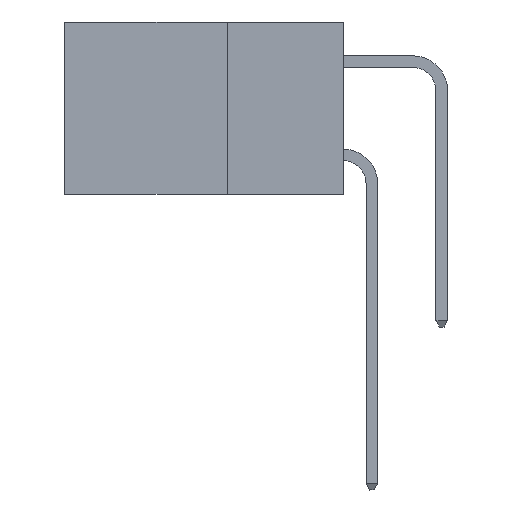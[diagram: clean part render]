
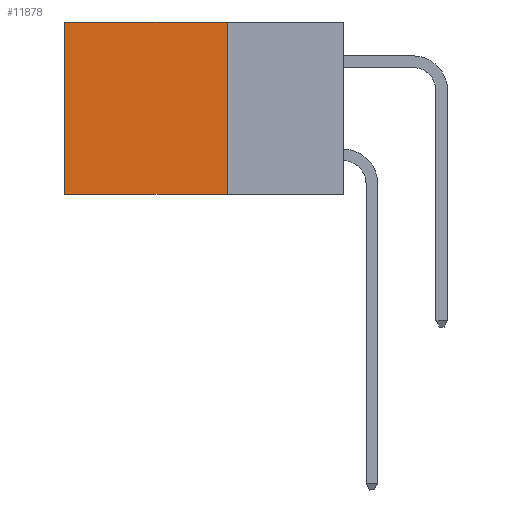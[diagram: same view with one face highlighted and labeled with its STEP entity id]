
A CAD part, left-side view. The second image highlights one B-rep face of the part: STEP entity #11878.
In plain terms, the highlighted planar face has unit normal (-1, 0, 0).
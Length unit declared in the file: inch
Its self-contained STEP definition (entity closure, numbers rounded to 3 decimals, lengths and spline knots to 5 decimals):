
#18 = LINE ( 'NONE', #16242, #24884 ) ;
#722 = ORIENTED_EDGE ( 'NONE', *, *, #7948, .F. ) ;
#1176 = EDGE_CURVE ( 'NONE', #22438, #4919, #18, .T. ) ;
#4236 = LINE ( 'NONE', #7374, #10094 ) ;
#4919 = VERTEX_POINT ( 'NONE', #7055 ) ;
#6580 = PLANE ( 'NONE',  #23420 ) ;
#6686 = CARTESIAN_POINT ( 'NONE',  ( 0.2615, 0.25, -0.37 ) ) ;
#7055 = CARTESIAN_POINT ( 'NONE',  ( 0.2615, 0.6, 0. ) ) ;
#7374 = CARTESIAN_POINT ( 'NONE',  ( 0.2615, 0.25, -0.37 ) ) ;
#7934 = VECTOR ( 'NONE', #24106, 39.37008 ) ;
#7948 = EDGE_CURVE ( 'NONE', #22438, #12869, #22964, .T. ) ;
#8072 = EDGE_CURVE ( 'NONE', #12869, #18795, #4236, .T. ) ;
#9987 = EDGE_LOOP ( 'NONE', ( #24803, #12125, #722, #21244 ) ) ;
#10094 = VECTOR ( 'NONE', #19073, 39.37008 ) ;
#10492 = CARTESIAN_POINT ( 'NONE',  ( 0.2615, 0.25, -0.37 ) ) ;
#10593 = DIRECTION ( 'NONE',  ( 0., 0., -1. ) ) ;
#11878 = ADVANCED_FACE ( 'NONE', ( #19382 ), #6580, .F. ) ;
#12063 = CARTESIAN_POINT ( 'NONE',  ( 0.2615, 0.6, -0.37 ) ) ;
#12125 = ORIENTED_EDGE ( 'NONE', *, *, #8072, .F. ) ;
#12483 = DIRECTION ( 'NONE',  ( 0., 0., -1. ) ) ;
#12579 = VECTOR ( 'NONE', #10593, 39.37008 ) ;
#12869 = VERTEX_POINT ( 'NONE', #13557 ) ;
#13557 = CARTESIAN_POINT ( 'NONE',  ( 0.2615, 0.25, -0.37 ) ) ;
#15934 = DIRECTION ( 'NONE',  ( 0., 1., 0. ) ) ;
#16242 = CARTESIAN_POINT ( 'NONE',  ( 0.2615, 0.25, 0. ) ) ;
#18795 = VERTEX_POINT ( 'NONE', #12063 ) ;
#19073 = DIRECTION ( 'NONE',  ( 0., 1., 0. ) ) ;
#19382 = FACE_OUTER_BOUND ( 'NONE', #9987, .T. ) ;
#20184 = CARTESIAN_POINT ( 'NONE',  ( 0.2615, 0.6, -0.37 ) ) ;
#21244 = ORIENTED_EDGE ( 'NONE', *, *, #1176, .T. ) ;
#21426 = CARTESIAN_POINT ( 'NONE',  ( 0.2615, 0.25, 0. ) ) ;
#22438 = VERTEX_POINT ( 'NONE', #21426 ) ;
#22964 = LINE ( 'NONE', #6686, #12579 ) ;
#23420 = AXIS2_PLACEMENT_3D ( 'NONE', #10492, #24164, #12483 ) ;
#23522 = LINE ( 'NONE', #20184, #7934 ) ;
#24106 = DIRECTION ( 'NONE',  ( 0., 0., -1. ) ) ;
#24164 = DIRECTION ( 'NONE',  ( 1., 0., 0. ) ) ;
#24803 = ORIENTED_EDGE ( 'NONE', *, *, #25013, .T. ) ;
#24884 = VECTOR ( 'NONE', #15934, 39.37008 ) ;
#25013 = EDGE_CURVE ( 'NONE', #4919, #18795, #23522, .T. ) ;
